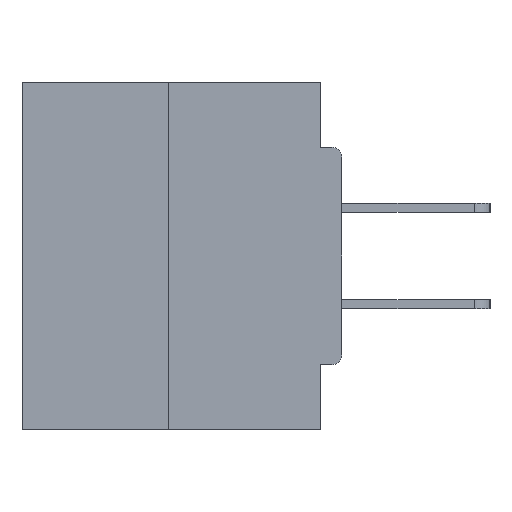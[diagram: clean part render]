
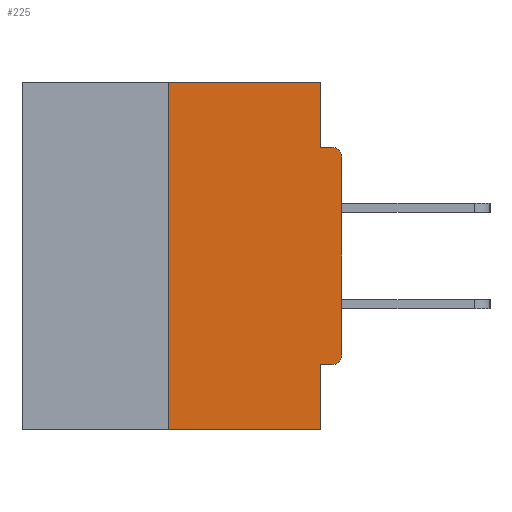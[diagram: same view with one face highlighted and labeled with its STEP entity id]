
A CAD part, left-side view. The second image highlights one B-rep face of the part: STEP entity #225.
In plain terms, the highlighted planar face has unit normal (-1, 0, 0).
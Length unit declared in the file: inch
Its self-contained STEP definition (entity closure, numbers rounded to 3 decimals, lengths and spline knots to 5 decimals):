
#225 = ADVANCED_FACE ( 'NONE', ( #32398 ), #19547, .F. ) ;
#243 = CARTESIAN_POINT ( 'NONE',  ( 0., 0.015, -0.3915 ) ) ;
#1274 = ORIENTED_EDGE ( 'NONE', *, *, #5931, .T. ) ;
#1377 = DIRECTION ( 'NONE',  ( 0., 0., 1. ) ) ;
#2152 = ORIENTED_EDGE ( 'NONE', *, *, #15195, .T. ) ;
#2165 = CARTESIAN_POINT ( 'NONE',  ( 0., 0.46, 0. ) ) ;
#2271 = CARTESIAN_POINT ( 'NONE',  ( 0., 0.031, -0.5 ) ) ;
#2665 = CARTESIAN_POINT ( 'NONE',  ( 0., 0.46, -0.5 ) ) ;
#3248 = EDGE_CURVE ( 'NONE', #16633, #21467, #32563, .T. ) ;
#3790 = LINE ( 'NONE', #6706, #6436 ) ;
#4072 = DIRECTION ( 'NONE',  ( -1., 0., 0. ) ) ;
#4112 = ORIENTED_EDGE ( 'NONE', *, *, #25375, .T. ) ;
#4155 = AXIS2_PLACEMENT_3D ( 'NONE', #6800, #4072, #8321 ) ;
#4211 = CARTESIAN_POINT ( 'NONE',  ( 0., 0., -0.3915 ) ) ;
#4273 = EDGE_CURVE ( 'NONE', #34597, #21608, #3790, .T. ) ;
#4385 = LINE ( 'NONE', #26524, #16177 ) ;
#4579 = EDGE_CURVE ( 'NONE', #19657, #8221, #29272, .T. ) ;
#4936 = EDGE_LOOP ( 'NONE', ( #12842, #16323, #2152, #30278, #19349, #4112, #1274, #17459, #28318, #24515 ) ) ;
#5025 = VERTEX_POINT ( 'NONE', #4211 ) ;
#5297 = CARTESIAN_POINT ( 'NONE',  ( 0., 0.46, 0. ) ) ;
#5501 = CARTESIAN_POINT ( 'NONE',  ( 0., 0.25, -0.5 ) ) ;
#5842 = DIRECTION ( 'NONE',  ( 0., 0., -1. ) ) ;
#5931 = EDGE_CURVE ( 'NONE', #5025, #19657, #12347, .T. ) ;
#6436 = VECTOR ( 'NONE', #17865, 39.37008 ) ;
#6503 = CARTESIAN_POINT ( 'NONE',  ( 0., 0., 0. ) ) ;
#6706 = CARTESIAN_POINT ( 'NONE',  ( 0., 0.031, -0.5 ) ) ;
#6800 = CARTESIAN_POINT ( 'NONE',  ( 0., 0.015, -0.1085 ) ) ;
#7105 = CARTESIAN_POINT ( 'NONE',  ( 0., 0.25, 0. ) ) ;
#7389 = VECTOR ( 'NONE', #15218, 39.37008 ) ;
#8221 = VERTEX_POINT ( 'NONE', #31541 ) ;
#8321 = DIRECTION ( 'NONE',  ( 0., 0., -1. ) ) ;
#8507 = CARTESIAN_POINT ( 'NONE',  ( 0., 0.031, -0.4065 ) ) ;
#9721 = LINE ( 'NONE', #18165, #7389 ) ;
#9726 = CARTESIAN_POINT ( 'NONE',  ( 0., 0.015, -0.4065 ) ) ;
#9830 = LINE ( 'NONE', #7105, #35626 ) ;
#10565 = DIRECTION ( 'NONE',  ( 0., -1., 0. ) ) ;
#10925 = CARTESIAN_POINT ( 'NONE',  ( 0., 0.25, 0. ) ) ;
#10942 = CARTESIAN_POINT ( 'NONE',  ( 0., 0., -0.1085 ) ) ;
#12347 = LINE ( 'NONE', #6503, #25234 ) ;
#12796 = CARTESIAN_POINT ( 'NONE',  ( 0., 0.031, -0.0935 ) ) ;
#12842 = ORIENTED_EDGE ( 'NONE', *, *, #3248, .F. ) ;
#13819 = DIRECTION ( 'NONE',  ( 0., -1., 0. ) ) ;
#15195 = EDGE_CURVE ( 'NONE', #21994, #21608, #27730, .T. ) ;
#15218 = DIRECTION ( 'NONE',  ( 0., 0., -1. ) ) ;
#15616 = CARTESIAN_POINT ( 'NONE',  ( 0., 0.031, 0. ) ) ;
#16177 = VECTOR ( 'NONE', #23601, 39.37008 ) ;
#16323 = ORIENTED_EDGE ( 'NONE', *, *, #27800, .F. ) ;
#16633 = VERTEX_POINT ( 'NONE', #10925 ) ;
#17459 = ORIENTED_EDGE ( 'NONE', *, *, #4579, .T. ) ;
#17865 = DIRECTION ( 'NONE',  ( 0., 0., -1. ) ) ;
#18029 = DIRECTION ( 'NONE',  ( 0., 1., 0. ) ) ;
#18165 = CARTESIAN_POINT ( 'NONE',  ( 0., 0.031, 0. ) ) ;
#19349 = ORIENTED_EDGE ( 'NONE', *, *, #21423, .F. ) ;
#19547 = PLANE ( 'NONE',  #33852 ) ;
#19657 = VERTEX_POINT ( 'NONE', #10942 ) ;
#20286 = VECTOR ( 'NONE', #10565, 39.37008 ) ;
#21013 = DIRECTION ( 'NONE',  ( 0., 0., 1. ) ) ;
#21423 = EDGE_CURVE ( 'NONE', #25610, #34597, #29537, .T. ) ;
#21467 = VERTEX_POINT ( 'NONE', #15616 ) ;
#21608 = VERTEX_POINT ( 'NONE', #2271 ) ;
#21994 = VERTEX_POINT ( 'NONE', #5501 ) ;
#22308 = VERTEX_POINT ( 'NONE', #12796 ) ;
#23601 = DIRECTION ( 'NONE',  ( 0., -1., 0. ) ) ;
#24515 = ORIENTED_EDGE ( 'NONE', *, *, #30453, .F. ) ;
#24604 = VECTOR ( 'NONE', #18029, 39.37008 ) ;
#24944 = DIRECTION ( 'NONE',  ( -1., 0., 0. ) ) ;
#25234 = VECTOR ( 'NONE', #1377, 39.37008 ) ;
#25375 = EDGE_CURVE ( 'NONE', #25610, #5025, #25901, .T. ) ;
#25610 = VERTEX_POINT ( 'NONE', #9726 ) ;
#25901 = CIRCLE ( 'NONE', #35268, 0.015 ) ;
#26524 = CARTESIAN_POINT ( 'NONE',  ( 0., 0., -0.0935 ) ) ;
#27730 = LINE ( 'NONE', #2665, #30445 ) ;
#27800 = EDGE_CURVE ( 'NONE', #21994, #16633, #9830, .T. ) ;
#28072 = DIRECTION ( 'NONE',  ( 0., 0., -1. ) ) ;
#28318 = ORIENTED_EDGE ( 'NONE', *, *, #31009, .F. ) ;
#29272 = CIRCLE ( 'NONE', #4155, 0.015 ) ;
#29537 = LINE ( 'NONE', #34696, #24604 ) ;
#30278 = ORIENTED_EDGE ( 'NONE', *, *, #4273, .F. ) ;
#30445 = VECTOR ( 'NONE', #13819, 39.37008 ) ;
#30453 = EDGE_CURVE ( 'NONE', #21467, #22308, #9721, .T. ) ;
#30539 = DIRECTION ( 'NONE',  ( 1., 0., 0. ) ) ;
#31009 = EDGE_CURVE ( 'NONE', #22308, #8221, #4385, .T. ) ;
#31541 = CARTESIAN_POINT ( 'NONE',  ( 0., 0.015, -0.0935 ) ) ;
#32398 = FACE_OUTER_BOUND ( 'NONE', #4936, .T. ) ;
#32563 = LINE ( 'NONE', #2165, #20286 ) ;
#33852 = AXIS2_PLACEMENT_3D ( 'NONE', #5297, #30539, #5842 ) ;
#34597 = VERTEX_POINT ( 'NONE', #8507 ) ;
#34696 = CARTESIAN_POINT ( 'NONE',  ( 0., 0., -0.4065 ) ) ;
#35268 = AXIS2_PLACEMENT_3D ( 'NONE', #243, #24944, #28072 ) ;
#35626 = VECTOR ( 'NONE', #21013, 39.37008 ) ;
